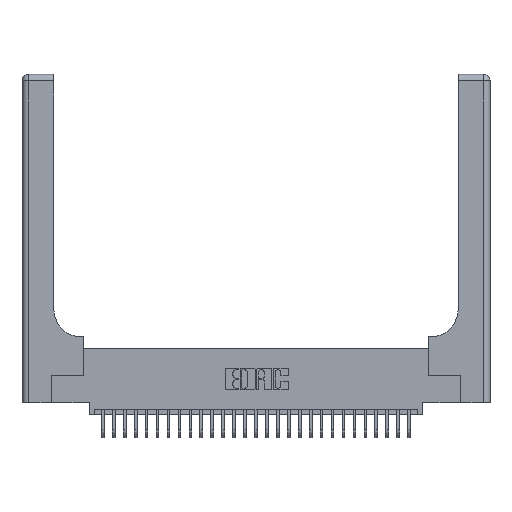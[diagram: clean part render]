
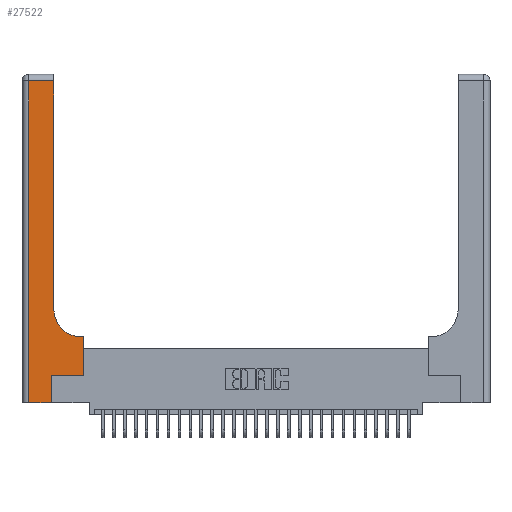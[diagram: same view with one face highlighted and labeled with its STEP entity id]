
A CAD part, top view. The second image highlights one B-rep face of the part: STEP entity #27522.
In plain terms, the highlighted planar face has unit normal (0, 0, 1).
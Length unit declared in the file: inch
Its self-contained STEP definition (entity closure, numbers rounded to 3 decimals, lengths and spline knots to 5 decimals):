
#91 = ORIENTED_EDGE ( 'NONE', *, *, #4143, .T. ) ;
#194 = CARTESIAN_POINT ( 'NONE',  ( 0.5415, 0.85, 0.37 ) ) ;
#340 = VERTEX_POINT ( 'NONE', #6990 ) ;
#352 = ORIENTED_EDGE ( 'NONE', *, *, #13732, .T. ) ;
#403 = DIRECTION ( 'NONE',  ( 0., 0., -1. ) ) ;
#1531 = DIRECTION ( 'NONE',  ( 1., 0., 0. ) ) ;
#2021 = CARTESIAN_POINT ( 'NONE',  ( 0., 2.94, 0.37 ) ) ;
#3106 = EDGE_CURVE ( 'NONE', #15537, #3767, #30784, .T. ) ;
#3461 = CARTESIAN_POINT ( 'NONE',  ( 0., 3., 0.37 ) ) ;
#3675 = CARTESIAN_POINT ( 'NONE',  ( 0.06, 0., 0.37 ) ) ;
#3767 = VERTEX_POINT ( 'NONE', #20884 ) ;
#4143 = EDGE_CURVE ( 'NONE', #340, #28776, #20039, .T. ) ;
#4406 = LINE ( 'NONE', #6156, #18058 ) ;
#4644 = DIRECTION ( 'NONE',  ( 0., 1., 0. ) ) ;
#4722 = AXIS2_PLACEMENT_3D ( 'NONE', #194, #403, #17080 ) ;
#4855 = VECTOR ( 'NONE', #12704, 39.37008 ) ;
#5014 = EDGE_CURVE ( 'NONE', #11570, #15537, #4406, .T. ) ;
#5142 = CARTESIAN_POINT ( 'NONE',  ( 0.2915, 0.6, 0.37 ) ) ;
#5406 = EDGE_CURVE ( 'NONE', #10994, #340, #20716, .T. ) ;
#5999 = PLANE ( 'NONE',  #19632 ) ;
#6156 = CARTESIAN_POINT ( 'NONE',  ( 0.269, 0., 0.37 ) ) ;
#6747 = CARTESIAN_POINT ( 'NONE',  ( 0.5415, 0.6, 0.37 ) ) ;
#6990 = CARTESIAN_POINT ( 'NONE',  ( 0.06, 2.94, 0.37 ) ) ;
#7293 = DIRECTION ( 'NONE',  ( -1., 0., 0. ) ) ;
#8084 = VECTOR ( 'NONE', #4644, 39.37008 ) ;
#8216 = LINE ( 'NONE', #5142, #8570 ) ;
#8260 = VECTOR ( 'NONE', #1531, 39.37008 ) ;
#8570 = VECTOR ( 'NONE', #19688, 39.37008 ) ;
#9905 = DIRECTION ( 'NONE',  ( 0., 1., 0. ) ) ;
#10000 = ORIENTED_EDGE ( 'NONE', *, *, #23785, .T. ) ;
#10013 = CARTESIAN_POINT ( 'NONE',  ( 0.2915, 2.94, 0.37 ) ) ;
#10628 = CIRCLE ( 'NONE', #4722, 0.25 ) ;
#10994 = VERTEX_POINT ( 'NONE', #10013 ) ;
#11492 = DIRECTION ( 'NONE',  ( 0., 1., 0. ) ) ;
#11570 = VERTEX_POINT ( 'NONE', #25597 ) ;
#11738 = CARTESIAN_POINT ( 'NONE',  ( 0.2915, 0.85, 0.37 ) ) ;
#12131 = VERTEX_POINT ( 'NONE', #15125 ) ;
#12314 = CARTESIAN_POINT ( 'NONE',  ( 0., 0., 0.37 ) ) ;
#12353 = VECTOR ( 'NONE', #7293, 39.37008 ) ;
#12595 = CARTESIAN_POINT ( 'NONE',  ( 0.06, 3., 0.37 ) ) ;
#12704 = DIRECTION ( 'NONE',  ( 0., -1., 0. ) ) ;
#12877 = CARTESIAN_POINT ( 'NONE',  ( 0.269, 0.25, 0.37 ) ) ;
#13090 = VERTEX_POINT ( 'NONE', #6747 ) ;
#13489 = CARTESIAN_POINT ( 'NONE',  ( 0.269, 0.25, 0.37 ) ) ;
#13732 = EDGE_CURVE ( 'NONE', #28776, #11570, #19134, .T. ) ;
#13844 = ORIENTED_EDGE ( 'NONE', *, *, #3106, .T. ) ;
#14824 = EDGE_CURVE ( 'NONE', #15168, #10994, #18869, .T. ) ;
#14859 = EDGE_CURVE ( 'NONE', #12131, #13090, #8216, .T. ) ;
#15125 = CARTESIAN_POINT ( 'NONE',  ( 0.5585, 0.6, 0.37 ) ) ;
#15168 = VERTEX_POINT ( 'NONE', #11738 ) ;
#15282 = ORIENTED_EDGE ( 'NONE', *, *, #16648, .T. ) ;
#15537 = VERTEX_POINT ( 'NONE', #12877 ) ;
#16648 = EDGE_CURVE ( 'NONE', #3767, #12131, #23312, .T. ) ;
#16785 = DIRECTION ( 'NONE',  ( 1., 0., 0. ) ) ;
#17080 = DIRECTION ( 'NONE',  ( 1., 0., 0. ) ) ;
#17150 = CARTESIAN_POINT ( 'NONE',  ( 0.2915, 3., 0.37 ) ) ;
#18058 = VECTOR ( 'NONE', #11492, 39.37008 ) ;
#18459 = ORIENTED_EDGE ( 'NONE', *, *, #14859, .T. ) ;
#18869 = LINE ( 'NONE', #17150, #25749 ) ;
#19134 = LINE ( 'NONE', #12314, #26731 ) ;
#19632 = AXIS2_PLACEMENT_3D ( 'NONE', #3461, #25369, #22973 ) ;
#19688 = DIRECTION ( 'NONE',  ( -1., 0., 0. ) ) ;
#19919 = EDGE_LOOP ( 'NONE', ( #30305, #21068, #91, #352, #27534, #13844, #15282, #18459, #10000 ) ) ;
#20039 = LINE ( 'NONE', #12595, #4855 ) ;
#20716 = LINE ( 'NONE', #2021, #12353 ) ;
#20884 = CARTESIAN_POINT ( 'NONE',  ( 0.5585, 0.25, 0.37 ) ) ;
#21068 = ORIENTED_EDGE ( 'NONE', *, *, #5406, .T. ) ;
#22973 = DIRECTION ( 'NONE',  ( -1., 0., 0. ) ) ;
#23312 = LINE ( 'NONE', #24315, #8084 ) ;
#23480 = FACE_OUTER_BOUND ( 'NONE', #19919, .T. ) ;
#23785 = EDGE_CURVE ( 'NONE', #13090, #15168, #10628, .T. ) ;
#24315 = CARTESIAN_POINT ( 'NONE',  ( 0.5585, 0.25, 0.37 ) ) ;
#25369 = DIRECTION ( 'NONE',  ( 0., 0., -1. ) ) ;
#25597 = CARTESIAN_POINT ( 'NONE',  ( 0.269, 0., 0.37 ) ) ;
#25749 = VECTOR ( 'NONE', #9905, 39.37008 ) ;
#26731 = VECTOR ( 'NONE', #16785, 39.37008 ) ;
#27522 = ADVANCED_FACE ( 'NONE', ( #23480 ), #5999, .F. ) ;
#27534 = ORIENTED_EDGE ( 'NONE', *, *, #5014, .T. ) ;
#28776 = VERTEX_POINT ( 'NONE', #3675 ) ;
#30305 = ORIENTED_EDGE ( 'NONE', *, *, #14824, .T. ) ;
#30784 = LINE ( 'NONE', #13489, #8260 ) ;
